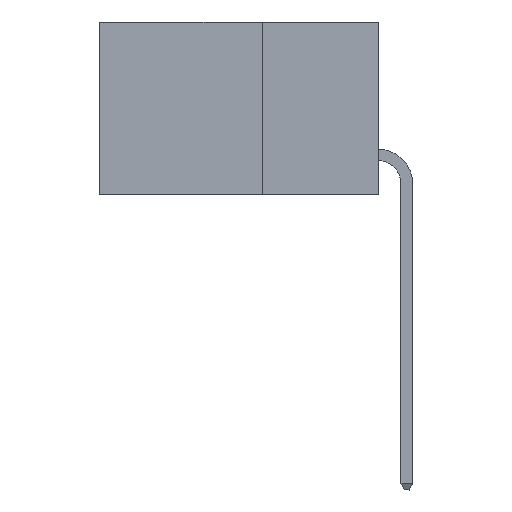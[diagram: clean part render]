
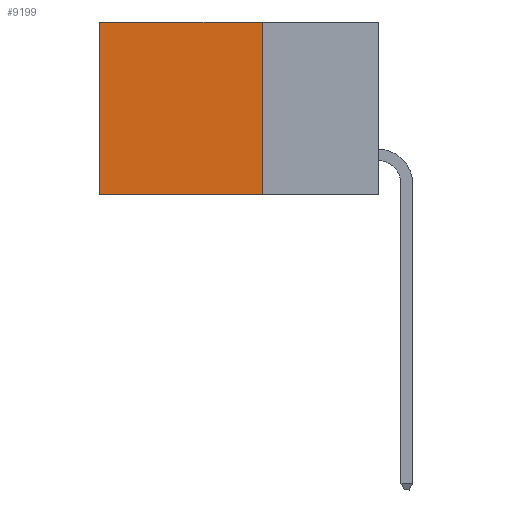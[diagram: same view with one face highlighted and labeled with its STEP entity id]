
A CAD part, left-side view. The second image highlights one B-rep face of the part: STEP entity #9199.
In plain terms, the highlighted planar face has unit normal (-1, 0, 0).
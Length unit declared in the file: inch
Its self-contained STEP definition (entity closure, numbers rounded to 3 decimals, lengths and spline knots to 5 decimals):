
#492 = PLANE ( 'NONE',  #8830 ) ;
#711 = EDGE_CURVE ( 'NONE', #5394, #7676, #9738, .T. ) ;
#1308 = VECTOR ( 'NONE', #6573, 39.37008 ) ;
#1816 = DIRECTION ( 'NONE',  ( 0., 0., -1. ) ) ;
#2855 = ORIENTED_EDGE ( 'NONE', *, *, #711, .T. ) ;
#3025 = ORIENTED_EDGE ( 'NONE', *, *, #5648, .F. ) ;
#3057 = VERTEX_POINT ( 'NONE', #7121 ) ;
#4353 = CARTESIAN_POINT ( 'NONE',  ( 0.298, 0.25, 0. ) ) ;
#4801 = LINE ( 'NONE', #8824, #1308 ) ;
#5359 = VERTEX_POINT ( 'NONE', #4353 ) ;
#5394 = VERTEX_POINT ( 'NONE', #8796 ) ;
#5598 = DIRECTION ( 'NONE',  ( 0., 0., -1. ) ) ;
#5648 = EDGE_CURVE ( 'NONE', #5359, #3057, #7682, .T. ) ;
#6142 = CARTESIAN_POINT ( 'NONE',  ( 0.298, 0.6, -0.37 ) ) ;
#6573 = DIRECTION ( 'NONE',  ( 0., 1., 0. ) ) ;
#6714 = VECTOR ( 'NONE', #5598, 39.37008 ) ;
#7121 = CARTESIAN_POINT ( 'NONE',  ( 0.298, 0.25, -0.37 ) ) ;
#7494 = EDGE_CURVE ( 'NONE', #5359, #5394, #10530, .T. ) ;
#7676 = VERTEX_POINT ( 'NONE', #6142 ) ;
#7682 = LINE ( 'NONE', #14517, #13517 ) ;
#8682 = ORIENTED_EDGE ( 'NONE', *, *, #7494, .T. ) ;
#8728 = DIRECTION ( 'NONE',  ( 1., 0., 0. ) ) ;
#8796 = CARTESIAN_POINT ( 'NONE',  ( 0.298, 0.6, 0. ) ) ;
#8824 = CARTESIAN_POINT ( 'NONE',  ( 0.298, 0.25, -0.37 ) ) ;
#8830 = AXIS2_PLACEMENT_3D ( 'NONE', #14111, #8728, #1816 ) ;
#9101 = CARTESIAN_POINT ( 'NONE',  ( 0.298, 0.6, 0. ) ) ;
#9199 = ADVANCED_FACE ( 'NONE', ( #12523 ), #492, .F. ) ;
#9200 = DIRECTION ( 'NONE',  ( 0., 0., -1. ) ) ;
#9738 = LINE ( 'NONE', #9101, #6714 ) ;
#10530 = LINE ( 'NONE', #14371, #13041 ) ;
#12523 = FACE_OUTER_BOUND ( 'NONE', #13114, .T. ) ;
#13041 = VECTOR ( 'NONE', #13339, 39.37008 ) ;
#13114 = EDGE_LOOP ( 'NONE', ( #2855, #14591, #3025, #8682 ) ) ;
#13125 = EDGE_CURVE ( 'NONE', #3057, #7676, #4801, .T. ) ;
#13339 = DIRECTION ( 'NONE',  ( 0., 1., 0. ) ) ;
#13517 = VECTOR ( 'NONE', #9200, 39.37008 ) ;
#14111 = CARTESIAN_POINT ( 'NONE',  ( 0.298, 0.25, 0. ) ) ;
#14371 = CARTESIAN_POINT ( 'NONE',  ( 0.298, 0.25, 0. ) ) ;
#14517 = CARTESIAN_POINT ( 'NONE',  ( 0.298, 0.25, 0. ) ) ;
#14591 = ORIENTED_EDGE ( 'NONE', *, *, #13125, .F. ) ;
